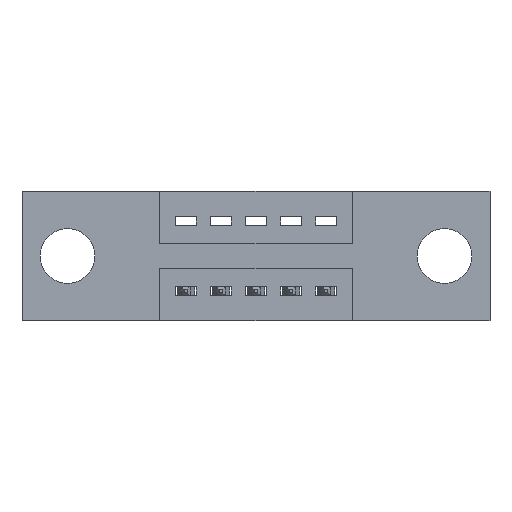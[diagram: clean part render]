
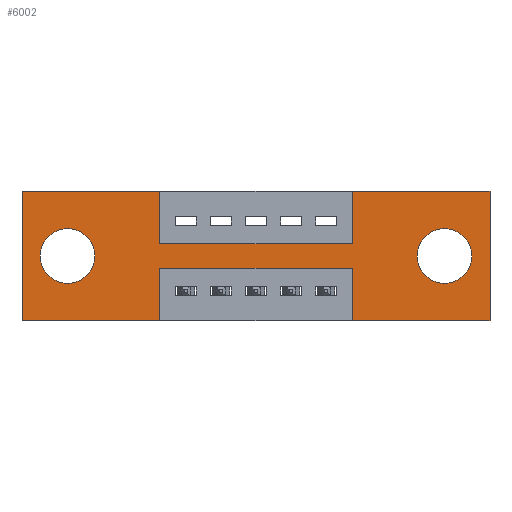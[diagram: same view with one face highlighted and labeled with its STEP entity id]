
A CAD part, front view. The second image highlights one B-rep face of the part: STEP entity #6002.
In plain terms, the highlighted planar face has unit normal (0, -1, 0).
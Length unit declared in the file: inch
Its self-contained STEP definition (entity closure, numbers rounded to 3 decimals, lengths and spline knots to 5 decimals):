
#19 = LINE ( 'NONE', #4347, #7911 ) ;
#94 = ORIENTED_EDGE ( 'NONE', *, *, #8258, .F. ) ;
#173 = AXIS2_PLACEMENT_3D ( 'NONE', #1900, #8624, #1136 ) ;
#286 = VERTEX_POINT ( 'NONE', #3531 ) ;
#349 = EDGE_CURVE ( 'NONE', #286, #1094, #1584, .T. ) ;
#395 = ORIENTED_EDGE ( 'NONE', *, *, #1570, .T. ) ;
#416 = EDGE_CURVE ( 'NONE', #5754, #6809, #2559, .T. ) ;
#446 = DIRECTION ( 'NONE',  ( 0., 0., 1. ) ) ;
#533 = CIRCLE ( 'NONE', #6570, 0.078 ) ;
#592 = CARTESIAN_POINT ( 'NONE',  ( 0., 0., 0. ) ) ;
#626 = DIRECTION ( 'NONE',  ( 0., 0., 1. ) ) ;
#749 = LINE ( 'NONE', #4509, #4434 ) ;
#751 = ORIENTED_EDGE ( 'NONE', *, *, #7168, .F. ) ;
#796 = DIRECTION ( 'NONE',  ( -1., 0., 0. ) ) ;
#808 = CIRCLE ( 'NONE', #173, 0.078 ) ;
#829 = CARTESIAN_POINT ( 'NONE',  ( 0.9425, 0., -0.15 ) ) ;
#854 = ORIENTED_EDGE ( 'NONE', *, *, #2035, .F. ) ;
#1059 = DIRECTION ( 'NONE',  ( 0., 0., 1. ) ) ;
#1094 = VERTEX_POINT ( 'NONE', #6606 ) ;
#1136 = DIRECTION ( 'NONE',  ( 0., 0., 1. ) ) ;
#1342 = DIRECTION ( 'NONE',  ( 1., 0., 0. ) ) ;
#1367 = CARTESIAN_POINT ( 'NONE',  ( 0.13, 0., -0.263 ) ) ;
#1467 = EDGE_CURVE ( 'NONE', #3776, #7662, #749, .T. ) ;
#1570 = EDGE_CURVE ( 'NONE', #4945, #4940, #2549, .T. ) ;
#1575 = EDGE_CURVE ( 'NONE', #4940, #4945, #533, .T. ) ;
#1584 = LINE ( 'NONE', #3559, #7555 ) ;
#1608 = LINE ( 'NONE', #3802, #7571 ) ;
#1645 = EDGE_CURVE ( 'NONE', #8187, #286, #2950, .T. ) ;
#1684 = VERTEX_POINT ( 'NONE', #8268 ) ;
#1697 = VERTEX_POINT ( 'NONE', #829 ) ;
#1807 = ORIENTED_EDGE ( 'NONE', *, *, #1467, .F. ) ;
#1900 = CARTESIAN_POINT ( 'NONE',  ( 0.13, 0., -0.185 ) ) ;
#1911 = CARTESIAN_POINT ( 'NONE',  ( 1.205, 0., -0.185 ) ) ;
#2024 = EDGE_CURVE ( 'NONE', #2636, #1684, #7313, .T. ) ;
#2034 = LINE ( 'NONE', #6716, #3222 ) ;
#2035 = EDGE_CURVE ( 'NONE', #6564, #2751, #4542, .T. ) ;
#2136 = ORIENTED_EDGE ( 'NONE', *, *, #8042, .F. ) ;
#2271 = VECTOR ( 'NONE', #5098, 39.37008 ) ;
#2496 = VERTEX_POINT ( 'NONE', #3654 ) ;
#2533 = CARTESIAN_POINT ( 'NONE',  ( 1.205, 0., -0.263 ) ) ;
#2549 = CIRCLE ( 'NONE', #5541, 0.078 ) ;
#2556 = DIRECTION ( 'NONE',  ( -1., 0., 0. ) ) ;
#2559 = CIRCLE ( 'NONE', #6048, 0.078 ) ;
#2619 = AXIS2_PLACEMENT_3D ( 'NONE', #7198, #8480, #6511 ) ;
#2636 = VERTEX_POINT ( 'NONE', #6092 ) ;
#2751 = VERTEX_POINT ( 'NONE', #4109 ) ;
#2780 = CARTESIAN_POINT ( 'NONE',  ( 1.205, 0., -0.107 ) ) ;
#2794 = DIRECTION ( 'NONE',  ( 0., 0., -1. ) ) ;
#2950 = LINE ( 'NONE', #6897, #7421 ) ;
#3067 = ORIENTED_EDGE ( 'NONE', *, *, #5939, .T. ) ;
#3162 = VECTOR ( 'NONE', #2794, 39.37008 ) ;
#3171 = DIRECTION ( 'NONE',  ( 0., 0., -1. ) ) ;
#3222 = VECTOR ( 'NONE', #1342, 39.37008 ) ;
#3307 = CARTESIAN_POINT ( 'NONE',  ( 0.9425, 0., -0.37 ) ) ;
#3531 = CARTESIAN_POINT ( 'NONE',  ( 0.9425, 0., -0.22 ) ) ;
#3559 = CARTESIAN_POINT ( 'NONE',  ( 0.3925, 0., -0.22 ) ) ;
#3654 = CARTESIAN_POINT ( 'NONE',  ( 0.9425, 0., 0. ) ) ;
#3776 = VERTEX_POINT ( 'NONE', #4778 ) ;
#3802 = CARTESIAN_POINT ( 'NONE',  ( 0.9425, 0., 0. ) ) ;
#3969 = ORIENTED_EDGE ( 'NONE', *, *, #6673, .F. ) ;
#4069 = LINE ( 'NONE', #592, #4613 ) ;
#4082 = CARTESIAN_POINT ( 'NONE',  ( 0., 0., -0.37 ) ) ;
#4109 = CARTESIAN_POINT ( 'NONE',  ( 0.3925, 0., 0. ) ) ;
#4110 = EDGE_LOOP ( 'NONE', ( #3067, #4324 ) ) ;
#4148 = DIRECTION ( 'NONE',  ( 0., 0., 1. ) ) ;
#4249 = CARTESIAN_POINT ( 'NONE',  ( 0.13, 0., -0.107 ) ) ;
#4296 = ORIENTED_EDGE ( 'NONE', *, *, #2024, .F. ) ;
#4324 = ORIENTED_EDGE ( 'NONE', *, *, #416, .T. ) ;
#4347 = CARTESIAN_POINT ( 'NONE',  ( 0.3925, 0., -0.37 ) ) ;
#4419 = CARTESIAN_POINT ( 'NONE',  ( 0.3925, 0., -0.15 ) ) ;
#4424 = CARTESIAN_POINT ( 'NONE',  ( 1.335, 0., 0. ) ) ;
#4434 = VECTOR ( 'NONE', #2556, 39.37008 ) ;
#4509 = CARTESIAN_POINT ( 'NONE',  ( 0., 0., -0.37 ) ) ;
#4534 = EDGE_CURVE ( 'NONE', #1094, #3776, #19, .T. ) ;
#4542 = LINE ( 'NONE', #4658, #5934 ) ;
#4611 = FACE_BOUND ( 'NONE', #6857, .T. ) ;
#4613 = VECTOR ( 'NONE', #626, 39.37008 ) ;
#4638 = VECTOR ( 'NONE', #5811, 39.37008 ) ;
#4658 = CARTESIAN_POINT ( 'NONE',  ( 0., 0., 0. ) ) ;
#4712 = EDGE_LOOP ( 'NONE', ( #5390, #7138, #8033, #751, #4296, #94, #2136, #6686, #7034, #854, #3969, #1807 ) ) ;
#4778 = CARTESIAN_POINT ( 'NONE',  ( 0.3925, 0., -0.37 ) ) ;
#4914 = CARTESIAN_POINT ( 'NONE',  ( 0.3925, 0., 0. ) ) ;
#4940 = VERTEX_POINT ( 'NONE', #2533 ) ;
#4945 = VERTEX_POINT ( 'NONE', #2780 ) ;
#5052 = CARTESIAN_POINT ( 'NONE',  ( 0., 0., 0. ) ) ;
#5098 = DIRECTION ( 'NONE',  ( 1., 0., 0. ) ) ;
#5186 = EDGE_CURVE ( 'NONE', #2751, #7792, #8560, .T. ) ;
#5293 = DIRECTION ( 'NONE',  ( 0., 0., -1. ) ) ;
#5390 = ORIENTED_EDGE ( 'NONE', *, *, #4534, .F. ) ;
#5452 = LINE ( 'NONE', #4082, #5999 ) ;
#5541 = AXIS2_PLACEMENT_3D ( 'NONE', #8016, #5877, #3171 ) ;
#5754 = VERTEX_POINT ( 'NONE', #1367 ) ;
#5763 = PLANE ( 'NONE',  #2619 ) ;
#5811 = DIRECTION ( 'NONE',  ( 0., 0., -1. ) ) ;
#5877 = DIRECTION ( 'NONE',  ( 0., 1., 0. ) ) ;
#5934 = VECTOR ( 'NONE', #5981, 39.37008 ) ;
#5939 = EDGE_CURVE ( 'NONE', #6809, #5754, #808, .T. ) ;
#5961 = DIRECTION ( 'NONE',  ( 0., 1., 0. ) ) ;
#5981 = DIRECTION ( 'NONE',  ( 1., 0., 0. ) ) ;
#5999 = VECTOR ( 'NONE', #8061, 39.37008 ) ;
#6002 = ADVANCED_FACE ( 'NONE', ( #4611, #8030, #8337 ), #5763, .T. ) ;
#6025 = CARTESIAN_POINT ( 'NONE',  ( 0.3925, 0., -0.15 ) ) ;
#6048 = AXIS2_PLACEMENT_3D ( 'NONE', #7234, #6486, #1059 ) ;
#6092 = CARTESIAN_POINT ( 'NONE',  ( 1.335, 0., 0. ) ) ;
#6486 = DIRECTION ( 'NONE',  ( 0., 1., 0. ) ) ;
#6492 = EDGE_CURVE ( 'NONE', #7792, #1697, #7484, .T. ) ;
#6511 = DIRECTION ( 'NONE',  ( 0., 0., -1. ) ) ;
#6564 = VERTEX_POINT ( 'NONE', #5052 ) ;
#6570 = AXIS2_PLACEMENT_3D ( 'NONE', #1911, #5961, #5293 ) ;
#6606 = CARTESIAN_POINT ( 'NONE',  ( 0.3925, 0., -0.22 ) ) ;
#6673 = EDGE_CURVE ( 'NONE', #7662, #6564, #4069, .T. ) ;
#6686 = ORIENTED_EDGE ( 'NONE', *, *, #6492, .F. ) ;
#6716 = CARTESIAN_POINT ( 'NONE',  ( 0., 0., 0. ) ) ;
#6809 = VERTEX_POINT ( 'NONE', #4249 ) ;
#6857 = EDGE_LOOP ( 'NONE', ( #395, #7478 ) ) ;
#6897 = CARTESIAN_POINT ( 'NONE',  ( 0.9425, 0., -0.37 ) ) ;
#7034 = ORIENTED_EDGE ( 'NONE', *, *, #5186, .F. ) ;
#7138 = ORIENTED_EDGE ( 'NONE', *, *, #349, .F. ) ;
#7168 = EDGE_CURVE ( 'NONE', #1684, #8187, #5452, .T. ) ;
#7198 = CARTESIAN_POINT ( 'NONE',  ( 0., 0., -0.37 ) ) ;
#7234 = CARTESIAN_POINT ( 'NONE',  ( 0.13, 0., -0.185 ) ) ;
#7313 = LINE ( 'NONE', #4424, #4638 ) ;
#7421 = VECTOR ( 'NONE', #4148, 39.37008 ) ;
#7478 = ORIENTED_EDGE ( 'NONE', *, *, #1575, .T. ) ;
#7484 = LINE ( 'NONE', #4419, #2271 ) ;
#7555 = VECTOR ( 'NONE', #796, 39.37008 ) ;
#7571 = VECTOR ( 'NONE', #446, 39.37008 ) ;
#7662 = VERTEX_POINT ( 'NONE', #8466 ) ;
#7725 = DIRECTION ( 'NONE',  ( 0., 0., -1. ) ) ;
#7792 = VERTEX_POINT ( 'NONE', #6025 ) ;
#7911 = VECTOR ( 'NONE', #7725, 39.37008 ) ;
#8016 = CARTESIAN_POINT ( 'NONE',  ( 1.205, 0., -0.185 ) ) ;
#8030 = FACE_BOUND ( 'NONE', #4110, .T. ) ;
#8033 = ORIENTED_EDGE ( 'NONE', *, *, #1645, .F. ) ;
#8042 = EDGE_CURVE ( 'NONE', #1697, #2496, #1608, .T. ) ;
#8061 = DIRECTION ( 'NONE',  ( -1., 0., 0. ) ) ;
#8187 = VERTEX_POINT ( 'NONE', #3307 ) ;
#8258 = EDGE_CURVE ( 'NONE', #2496, #2636, #2034, .T. ) ;
#8268 = CARTESIAN_POINT ( 'NONE',  ( 1.335, 0., -0.37 ) ) ;
#8337 = FACE_OUTER_BOUND ( 'NONE', #4712, .T. ) ;
#8466 = CARTESIAN_POINT ( 'NONE',  ( 0., 0., -0.37 ) ) ;
#8480 = DIRECTION ( 'NONE',  ( 0., -1., 0. ) ) ;
#8560 = LINE ( 'NONE', #4914, #3162 ) ;
#8624 = DIRECTION ( 'NONE',  ( 0., 1., 0. ) ) ;
